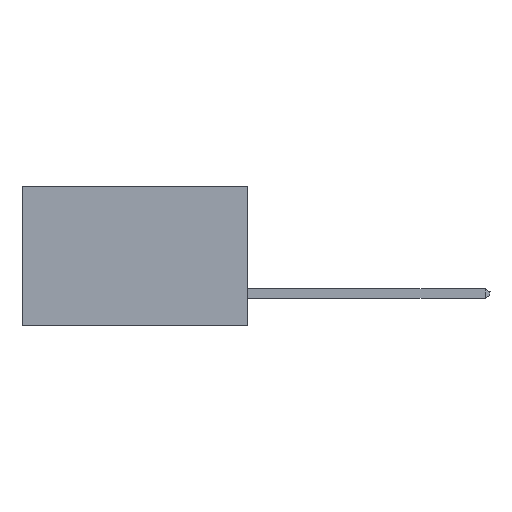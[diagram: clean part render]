
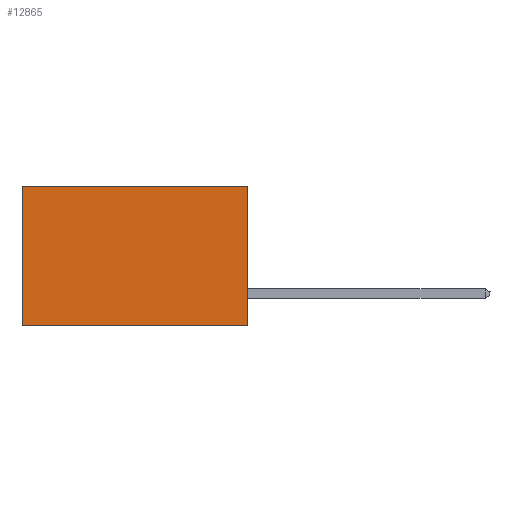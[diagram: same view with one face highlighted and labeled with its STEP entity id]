
A CAD part, left-side view. The second image highlights one B-rep face of the part: STEP entity #12865.
In plain terms, the highlighted planar face has unit normal (-1, 0, 0).
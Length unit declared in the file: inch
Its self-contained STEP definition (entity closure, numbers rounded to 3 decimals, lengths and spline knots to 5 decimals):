
#173 = CARTESIAN_POINT ( 'NONE',  ( 0.298, 0., 0. ) ) ;
#352 = CARTESIAN_POINT ( 'NONE',  ( 0.298, 0.6, 0. ) ) ;
#395 = FACE_OUTER_BOUND ( 'NONE', #9148, .T. ) ;
#850 = VECTOR ( 'NONE', #6347, 39.37008 ) ;
#860 = EDGE_CURVE ( 'NONE', #11046, #4156, #3892, .T. ) ;
#943 = VECTOR ( 'NONE', #5826, 39.37008 ) ;
#1674 = DIRECTION ( 'NONE',  ( 0., 0., -1. ) ) ;
#1765 = VECTOR ( 'NONE', #12593, 39.37008 ) ;
#2011 = VERTEX_POINT ( 'NONE', #10465 ) ;
#3846 = CARTESIAN_POINT ( 'NONE',  ( 0.298, 0.6, 0. ) ) ;
#3863 = ORIENTED_EDGE ( 'NONE', *, *, #10484, .F. ) ;
#3892 = LINE ( 'NONE', #352, #12318 ) ;
#4156 = VERTEX_POINT ( 'NONE', #14270 ) ;
#4721 = LINE ( 'NONE', #173, #1765 ) ;
#4751 = EDGE_CURVE ( 'NONE', #2011, #7875, #4721, .T. ) ;
#5427 = CARTESIAN_POINT ( 'NONE',  ( 0.298, 0., -0.37 ) ) ;
#5826 = DIRECTION ( 'NONE',  ( 0., 1., 0. ) ) ;
#6347 = DIRECTION ( 'NONE',  ( 0., 1., 0. ) ) ;
#7426 = AXIS2_PLACEMENT_3D ( 'NONE', #12706, #9104, #15379 ) ;
#7875 = VERTEX_POINT ( 'NONE', #5427 ) ;
#8142 = EDGE_CURVE ( 'NONE', #2011, #11046, #9398, .T. ) ;
#8348 = CARTESIAN_POINT ( 'NONE',  ( 0.298, 0., 0. ) ) ;
#9104 = DIRECTION ( 'NONE',  ( 1., 0., 0. ) ) ;
#9148 = EDGE_LOOP ( 'NONE', ( #15451, #3863, #15898, #14926 ) ) ;
#9398 = LINE ( 'NONE', #8348, #943 ) ;
#10465 = CARTESIAN_POINT ( 'NONE',  ( 0.298, 0., 0. ) ) ;
#10484 = EDGE_CURVE ( 'NONE', #7875, #4156, #15555, .T. ) ;
#11046 = VERTEX_POINT ( 'NONE', #3846 ) ;
#12318 = VECTOR ( 'NONE', #1674, 39.37008 ) ;
#12593 = DIRECTION ( 'NONE',  ( 0., 0., -1. ) ) ;
#12605 = CARTESIAN_POINT ( 'NONE',  ( 0.298, 0., -0.37 ) ) ;
#12706 = CARTESIAN_POINT ( 'NONE',  ( 0.298, 0., 0. ) ) ;
#12865 = ADVANCED_FACE ( 'NONE', ( #395 ), #13917, .F. ) ;
#13917 = PLANE ( 'NONE',  #7426 ) ;
#14270 = CARTESIAN_POINT ( 'NONE',  ( 0.298, 0.6, -0.37 ) ) ;
#14926 = ORIENTED_EDGE ( 'NONE', *, *, #8142, .T. ) ;
#15379 = DIRECTION ( 'NONE',  ( 0., 0., -1. ) ) ;
#15451 = ORIENTED_EDGE ( 'NONE', *, *, #860, .T. ) ;
#15555 = LINE ( 'NONE', #12605, #850 ) ;
#15898 = ORIENTED_EDGE ( 'NONE', *, *, #4751, .F. ) ;
